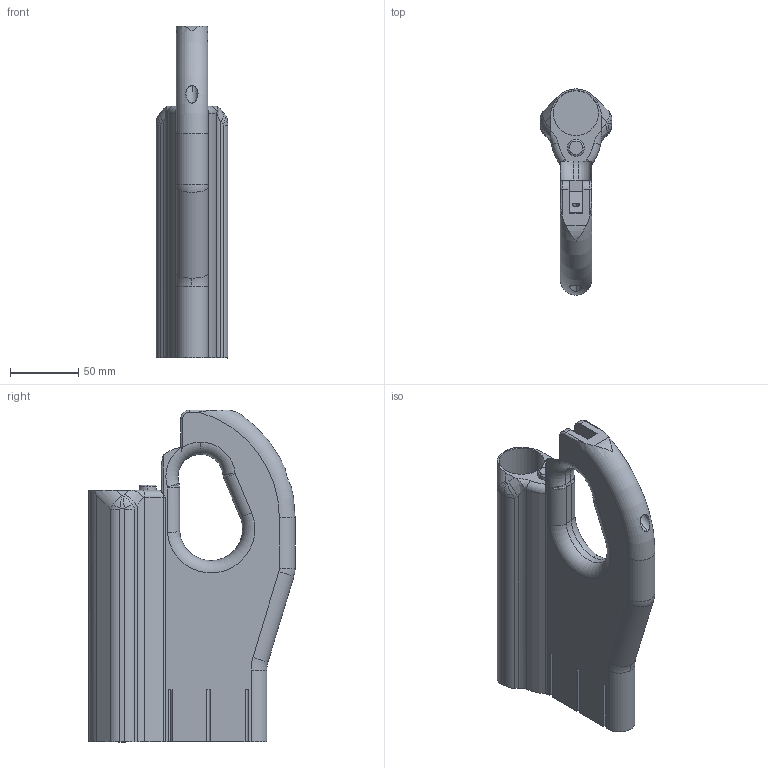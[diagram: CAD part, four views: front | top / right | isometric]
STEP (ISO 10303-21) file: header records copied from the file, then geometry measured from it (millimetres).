
FILE_DESCRIPTION (( 'STEP AP214' ), '1' );
FILE_NAME ('P-15_V2.STEP', '2013-12-11T21:46:24', ( 'elpi' ), ( '' ), 'SwSTEP 2.0', 'SolidWorks 2013', '' );
FILE_SCHEMA (( 'AUTOMOTIVE_DESIGN' ));
Length unit declared in the file: inch
Products named in the file (1): P-15_V2
Bounding box: 52.54 x 150.68 x 242.61 mm (x, y, z)
Volume: 474894.2 mm3; surface area: 119415.8 mm2
Topology: 1 solids, 1 shells, 167 faces, 441 edges, 275 vertices
Faces by surface type: cylinder 70, plane 51, torus 28, bspline 14, sphere 4
Entity records: 7545 total; most frequent: CARTESIAN_POINT 2271, ORIENTED_EDGE 866, DIRECTION 828, EDGE_CURVE 433, AXIS2_PLACEMENT_3D 319, VERTEX_POINT 275, VECTOR 190, LINE 190
